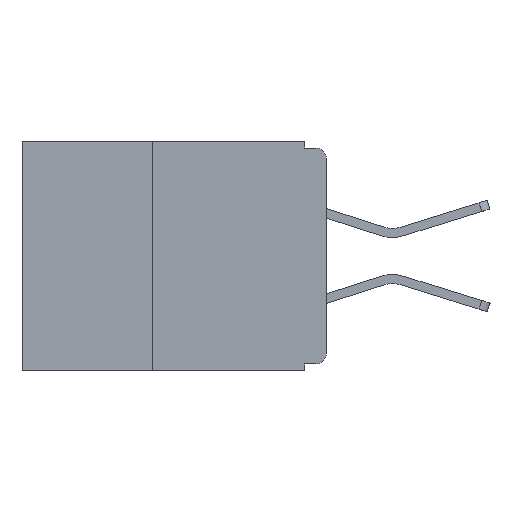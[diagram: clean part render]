
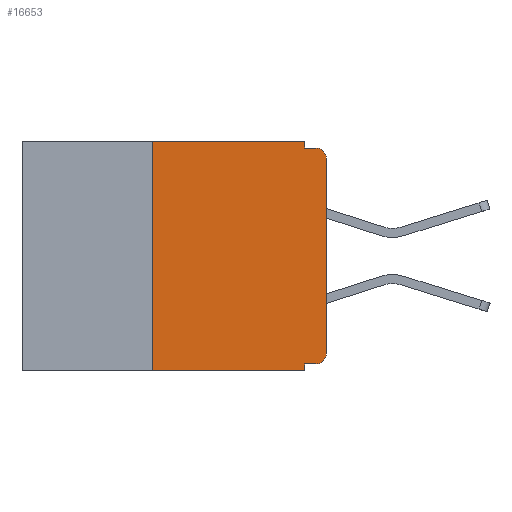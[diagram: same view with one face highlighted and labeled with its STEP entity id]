
A CAD part, left-side view. The second image highlights one B-rep face of the part: STEP entity #16653.
In plain terms, the highlighted planar face has unit normal (-1, 0, 0).
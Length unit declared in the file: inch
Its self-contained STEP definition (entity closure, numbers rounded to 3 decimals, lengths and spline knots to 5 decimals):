
#6 = ORIENTED_EDGE ( 'NONE', *, *, #5502, .F. ) ;
#481 = ORIENTED_EDGE ( 'NONE', *, *, #2580, .F. ) ;
#594 = EDGE_CURVE ( 'NONE', #7579, #10786, #16783, .T. ) ;
#1764 = VERTEX_POINT ( 'NONE', #10016 ) ;
#1891 = CARTESIAN_POINT ( 'NONE',  ( 0., 0.015, -0.305 ) ) ;
#2181 = CARTESIAN_POINT ( 'NONE',  ( 0., 0., -0.305 ) ) ;
#2417 = VERTEX_POINT ( 'NONE', #11279 ) ;
#2580 = EDGE_CURVE ( 'NONE', #7579, #9494, #16642, .T. ) ;
#2645 = ORIENTED_EDGE ( 'NONE', *, *, #9535, .T. ) ;
#2731 = DIRECTION ( 'NONE',  ( 0., 1., 0. ) ) ;
#2746 = DIRECTION ( 'NONE',  ( 1., 0., 0. ) ) ;
#2824 = DIRECTION ( 'NONE',  ( 0., 0., 1. ) ) ;
#2927 = DIRECTION ( 'NONE',  ( 0., 0., 1. ) ) ;
#3010 = CIRCLE ( 'NONE', #12756, 0.015 ) ;
#3362 = DIRECTION ( 'NONE',  ( 0., 0., -1. ) ) ;
#3472 = EDGE_CURVE ( 'NONE', #2417, #7428, #3010, .T. ) ;
#3893 = CARTESIAN_POINT ( 'NONE',  ( 0., 0.015, -0.32 ) ) ;
#3940 = CARTESIAN_POINT ( 'NONE',  ( 0., 0.25, -0.33 ) ) ;
#4618 = ORIENTED_EDGE ( 'NONE', *, *, #14299, .F. ) ;
#4649 = ORIENTED_EDGE ( 'NONE', *, *, #12577, .T. ) ;
#4664 = DIRECTION ( 'NONE',  ( 0., 0., -1. ) ) ;
#4757 = LINE ( 'NONE', #18692, #12900 ) ;
#5361 = DIRECTION ( 'NONE',  ( 0., 0., -1. ) ) ;
#5502 = EDGE_CURVE ( 'NONE', #1764, #17144, #16760, .T. ) ;
#5870 = CARTESIAN_POINT ( 'NONE',  ( 0., 0.437, 0. ) ) ;
#6647 = EDGE_LOOP ( 'NONE', ( #2645, #14674, #17364, #6, #4618, #481, #13905, #7108, #13231, #4649 ) ) ;
#7108 = ORIENTED_EDGE ( 'NONE', *, *, #16530, .F. ) ;
#7428 = VERTEX_POINT ( 'NONE', #10711 ) ;
#7579 = VERTEX_POINT ( 'NONE', #12486 ) ;
#7733 = VECTOR ( 'NONE', #18265, 39.37008 ) ;
#8216 = VERTEX_POINT ( 'NONE', #3893 ) ;
#8277 = AXIS2_PLACEMENT_3D ( 'NONE', #1891, #12059, #3362 ) ;
#8337 = EDGE_CURVE ( 'NONE', #8216, #10864, #11713, .T. ) ;
#8942 = EDGE_CURVE ( 'NONE', #17144, #7428, #16081, .T. ) ;
#9111 = VECTOR ( 'NONE', #14550, 39.37008 ) ;
#9494 = VERTEX_POINT ( 'NONE', #17199 ) ;
#9535 = EDGE_CURVE ( 'NONE', #14111, #2417, #4757, .T. ) ;
#10011 = AXIS2_PLACEMENT_3D ( 'NONE', #11434, #2746, #12891 ) ;
#10016 = CARTESIAN_POINT ( 'NONE',  ( 0., 0.031, 0. ) ) ;
#10711 = CARTESIAN_POINT ( 'NONE',  ( 0., 0.015, -0.01 ) ) ;
#10786 = VERTEX_POINT ( 'NONE', #13449 ) ;
#10792 = VECTOR ( 'NONE', #2731, 39.37008 ) ;
#10864 = VERTEX_POINT ( 'NONE', #12184 ) ;
#11279 = CARTESIAN_POINT ( 'NONE',  ( 0., 0., -0.025 ) ) ;
#11336 = VECTOR ( 'NONE', #15891, 39.37008 ) ;
#11413 = CIRCLE ( 'NONE', #8277, 0.015 ) ;
#11434 = CARTESIAN_POINT ( 'NONE',  ( 0., 0.437, 0. ) ) ;
#11713 = LINE ( 'NONE', #12872, #10792 ) ;
#12059 = DIRECTION ( 'NONE',  ( -1., 0., 0. ) ) ;
#12184 = CARTESIAN_POINT ( 'NONE',  ( 0., 0.031, -0.32 ) ) ;
#12462 = VECTOR ( 'NONE', #4664, 39.37008 ) ;
#12486 = CARTESIAN_POINT ( 'NONE',  ( 0., 0.25, -0.33 ) ) ;
#12577 = EDGE_CURVE ( 'NONE', #8216, #14111, #11413, .T. ) ;
#12578 = CARTESIAN_POINT ( 'NONE',  ( 0., 0.031, -0.33 ) ) ;
#12756 = AXIS2_PLACEMENT_3D ( 'NONE', #18395, #17978, #16680 ) ;
#12802 = VECTOR ( 'NONE', #2927, 39.37008 ) ;
#12872 = CARTESIAN_POINT ( 'NONE',  ( 0., 0., -0.32 ) ) ;
#12891 = DIRECTION ( 'NONE',  ( 0., 0., -1. ) ) ;
#12900 = VECTOR ( 'NONE', #2824, 39.37008 ) ;
#13024 = VECTOR ( 'NONE', #5361, 39.37008 ) ;
#13231 = ORIENTED_EDGE ( 'NONE', *, *, #8337, .F. ) ;
#13449 = CARTESIAN_POINT ( 'NONE',  ( 0., 0.031, -0.33 ) ) ;
#13905 = ORIENTED_EDGE ( 'NONE', *, *, #594, .T. ) ;
#14111 = VERTEX_POINT ( 'NONE', #2181 ) ;
#14299 = EDGE_CURVE ( 'NONE', #9494, #1764, #16351, .T. ) ;
#14380 = CARTESIAN_POINT ( 'NONE',  ( 0., 0., -0.01 ) ) ;
#14550 = DIRECTION ( 'NONE',  ( 0., -1., 0. ) ) ;
#14674 = ORIENTED_EDGE ( 'NONE', *, *, #3472, .T. ) ;
#14713 = CARTESIAN_POINT ( 'NONE',  ( 0., 0.031, 0. ) ) ;
#15399 = CARTESIAN_POINT ( 'NONE',  ( 0., 0.031, -0.01 ) ) ;
#15891 = DIRECTION ( 'NONE',  ( 0., -1., 0. ) ) ;
#16081 = LINE ( 'NONE', #14380, #11336 ) ;
#16351 = LINE ( 'NONE', #5870, #9111 ) ;
#16530 = EDGE_CURVE ( 'NONE', #10864, #10786, #16875, .T. ) ;
#16642 = LINE ( 'NONE', #3940, #12802 ) ;
#16653 = ADVANCED_FACE ( 'NONE', ( #18446 ), #18625, .F. ) ;
#16680 = DIRECTION ( 'NONE',  ( 0., 0., -1. ) ) ;
#16760 = LINE ( 'NONE', #14713, #12462 ) ;
#16783 = LINE ( 'NONE', #17981, #7733 ) ;
#16875 = LINE ( 'NONE', #12578, #13024 ) ;
#17144 = VERTEX_POINT ( 'NONE', #15399 ) ;
#17199 = CARTESIAN_POINT ( 'NONE',  ( 0., 0.25, 0. ) ) ;
#17364 = ORIENTED_EDGE ( 'NONE', *, *, #8942, .F. ) ;
#17978 = DIRECTION ( 'NONE',  ( -1., 0., 0. ) ) ;
#17981 = CARTESIAN_POINT ( 'NONE',  ( 0., 0.437, -0.33 ) ) ;
#18265 = DIRECTION ( 'NONE',  ( 0., -1., 0. ) ) ;
#18395 = CARTESIAN_POINT ( 'NONE',  ( 0., 0.015, -0.025 ) ) ;
#18446 = FACE_OUTER_BOUND ( 'NONE', #6647, .T. ) ;
#18625 = PLANE ( 'NONE',  #10011 ) ;
#18692 = CARTESIAN_POINT ( 'NONE',  ( 0., 0., 0. ) ) ;
